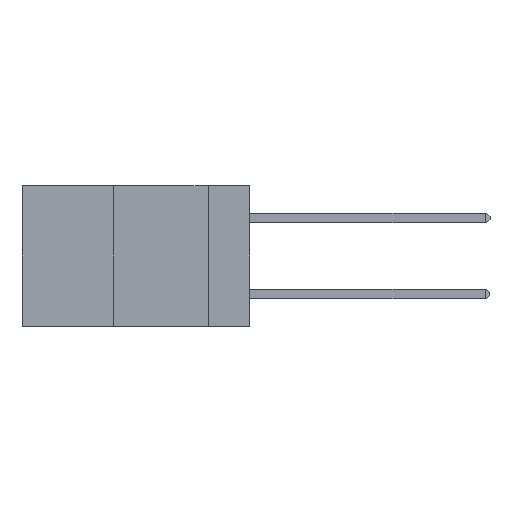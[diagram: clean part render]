
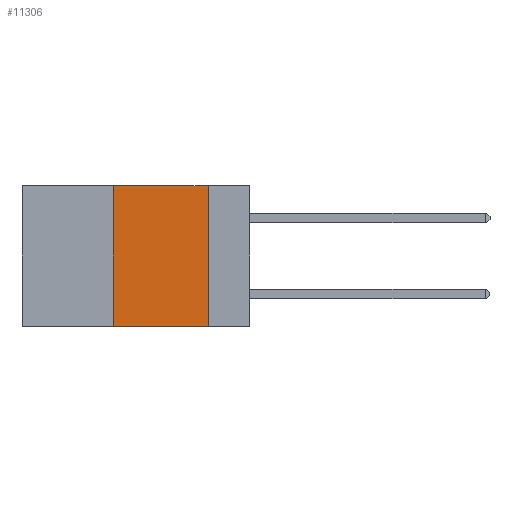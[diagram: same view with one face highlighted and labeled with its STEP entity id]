
A CAD part, left-side view. The second image highlights one B-rep face of the part: STEP entity #11306.
In plain terms, the highlighted planar face has unit normal (-1, 0, 0).
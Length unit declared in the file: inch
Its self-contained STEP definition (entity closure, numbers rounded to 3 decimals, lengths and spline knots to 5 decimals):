
#424 = CARTESIAN_POINT ( 'NONE',  ( 0., 0.11, -0.37 ) ) ;
#1354 = DIRECTION ( 'NONE',  ( 1., 0., 0. ) ) ;
#1594 = EDGE_CURVE ( 'NONE', #8173, #5840, #14734, .T. ) ;
#3200 = DIRECTION ( 'NONE',  ( 0., 0., -1. ) ) ;
#3730 = AXIS2_PLACEMENT_3D ( 'NONE', #13720, #1354, #10069 ) ;
#4116 = CARTESIAN_POINT ( 'NONE',  ( 0., 0.36, 0. ) ) ;
#4130 = VECTOR ( 'NONE', #10578, 39.37008 ) ;
#5840 = VERTEX_POINT ( 'NONE', #4116 ) ;
#6158 = DIRECTION ( 'NONE',  ( 0., -1., 0. ) ) ;
#6188 = CARTESIAN_POINT ( 'NONE',  ( 0., 0.36, 0. ) ) ;
#7868 = LINE ( 'NONE', #12962, #4130 ) ;
#7961 = VERTEX_POINT ( 'NONE', #424 ) ;
#8081 = LINE ( 'NONE', #10649, #11377 ) ;
#8173 = VERTEX_POINT ( 'NONE', #12183 ) ;
#8632 = CARTESIAN_POINT ( 'NONE',  ( 0., 0.6, -0.37 ) ) ;
#8816 = PLANE ( 'NONE',  #3730 ) ;
#8882 = EDGE_LOOP ( 'NONE', ( #12617, #12351, #11072, #10836 ) ) ;
#9118 = VECTOR ( 'NONE', #6158, 39.37008 ) ;
#10017 = EDGE_CURVE ( 'NONE', #8173, #7961, #11986, .T. ) ;
#10069 = DIRECTION ( 'NONE',  ( 0., 0., -1. ) ) ;
#10578 = DIRECTION ( 'NONE',  ( 0., -1., 0. ) ) ;
#10649 = CARTESIAN_POINT ( 'NONE',  ( 0., 0.11, 0. ) ) ;
#10836 = ORIENTED_EDGE ( 'NONE', *, *, #10017, .T. ) ;
#11072 = ORIENTED_EDGE ( 'NONE', *, *, #1594, .F. ) ;
#11306 = ADVANCED_FACE ( 'NONE', ( #12703 ), #8816, .F. ) ;
#11377 = VECTOR ( 'NONE', #3200, 39.37008 ) ;
#11597 = EDGE_CURVE ( 'NONE', #13336, #7961, #8081, .T. ) ;
#11805 = VECTOR ( 'NONE', #14891, 39.37008 ) ;
#11986 = LINE ( 'NONE', #8632, #9118 ) ;
#12183 = CARTESIAN_POINT ( 'NONE',  ( 0., 0.36, -0.37 ) ) ;
#12212 = EDGE_CURVE ( 'NONE', #5840, #13336, #7868, .T. ) ;
#12351 = ORIENTED_EDGE ( 'NONE', *, *, #12212, .F. ) ;
#12617 = ORIENTED_EDGE ( 'NONE', *, *, #11597, .F. ) ;
#12703 = FACE_OUTER_BOUND ( 'NONE', #8882, .T. ) ;
#12962 = CARTESIAN_POINT ( 'NONE',  ( 0., 0.6, 0. ) ) ;
#13336 = VERTEX_POINT ( 'NONE', #15919 ) ;
#13720 = CARTESIAN_POINT ( 'NONE',  ( 0., 0.6, 0. ) ) ;
#14734 = LINE ( 'NONE', #6188, #11805 ) ;
#14891 = DIRECTION ( 'NONE',  ( 0., 0., 1. ) ) ;
#15919 = CARTESIAN_POINT ( 'NONE',  ( 0., 0.11, 0. ) ) ;
